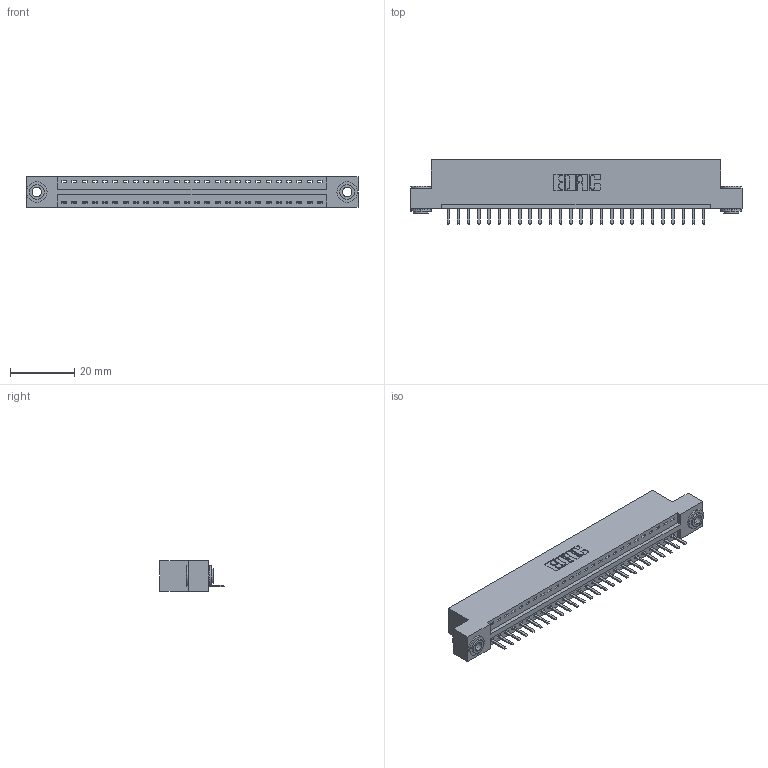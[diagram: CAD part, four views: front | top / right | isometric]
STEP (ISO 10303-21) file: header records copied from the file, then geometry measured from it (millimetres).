
FILE_DESCRIPTION (( 'STEP AP203' ), '1' );
FILE_NAME ('396-026-520-103.STEP', '2019-10-27T06:53:03', ( '' ), ( '' ), 'SwSTEP 2.0', 'SolidWorks 2016', '' );
FILE_SCHEMA (( 'CONFIG_CONTROL_DESIGN' ));
Length unit declared in the file: inch
Products named in the file (4): 345-250-002_345-250-002-102; 396-026-520-103; 345-292-001_345-293-120; 346 Part_Flush Mounting Lugs - 0.156 Dia-TH
Assembly tree (29 placements, depth 2):
  396-026-520-103
    346 Part_Flush Mounting Lugs - 0.156 Dia-TH
    345-292-001_345-293-120  x26
    345-250-002_345-250-002-102  x2
Bounding box: 103.12 x 20.02 x 9.4 mm (x, y, z)
Volume: 9705.6 mm3; surface area: 11927.6 mm2
Topology: 29 solids, 29 shells, 1772 faces, 5189 edges, 3386 vertices
Faces by surface type: plane 1178, cylinder 586, cone 8
Entity records: 19054 total; most frequent: CARTESIAN_POINT 3261, ORIENTED_EDGE 3202, DIRECTION 2915, EDGE_CURVE 1601, VECTOR 1337, LINE 1337, VERTEX_POINT 1062, AXIS2_PLACEMENT_3D 789
